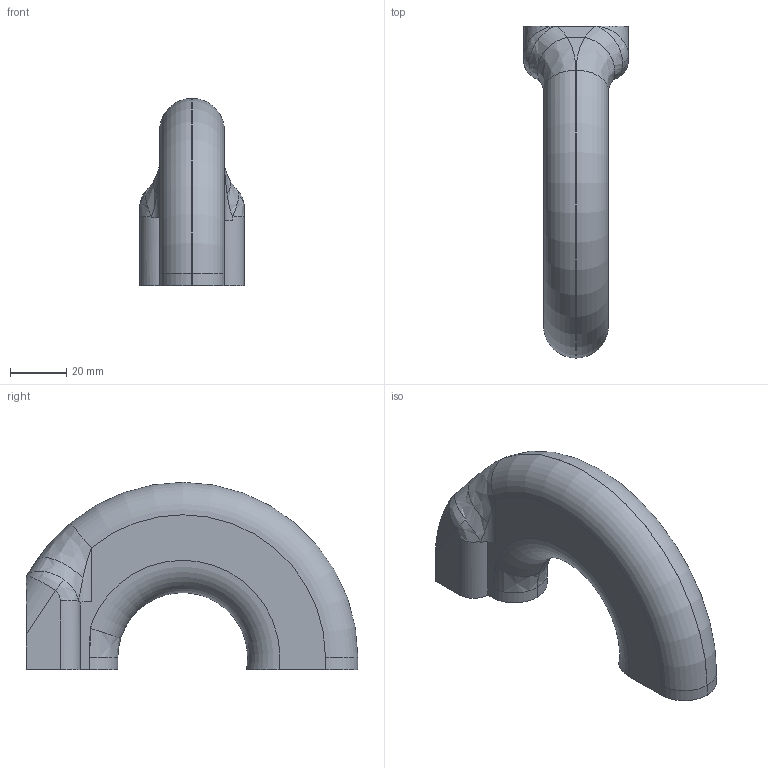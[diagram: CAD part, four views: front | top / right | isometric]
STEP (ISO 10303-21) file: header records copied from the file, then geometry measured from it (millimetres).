
FILE_DESCRIPTION (( 'STEP AP214' ), '1' );
FILE_NAME ('Unbuffered Pistol_2.STEP', '2013-09-01T16:58:21', ( 'Asher' ), ( '' ), 'SwSTEP 2.0', 'SolidWorks 2013', '' );
FILE_SCHEMA (( 'AUTOMOTIVE_DESIGN' ));
Length unit declared in the file: millimetre
Products named in the file (1): Unbuffered Pistol_2
Bounding box: 37.13 x 117.8 x 66.49 mm (x, y, z)
Volume: 119650.3 mm3; surface area: 17479.4 mm2
Topology: 1 solids, 1 shells, 45 faces, 113 edges, 68 vertices
Faces by surface type: cylinder 15, bspline 14, plane 12, torus 4
Entity records: 2167 total; most frequent: CARTESIAN_POINT 1159, ORIENTED_EDGE 222, DIRECTION 185, EDGE_CURVE 111, AXIS2_PLACEMENT_3D 72, VERTEX_POINT 68, ADVANCED_FACE 45, FACE_OUTER_BOUND 45
